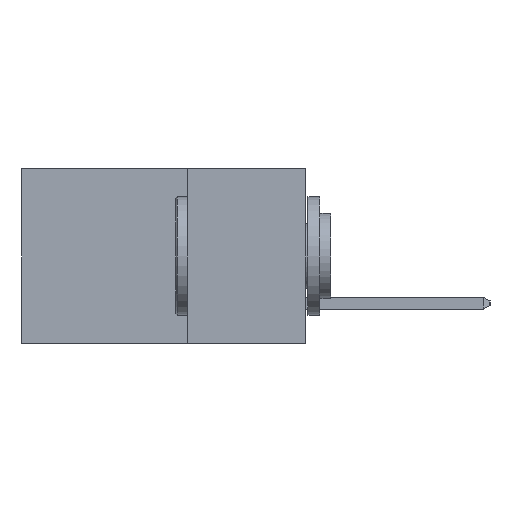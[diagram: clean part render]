
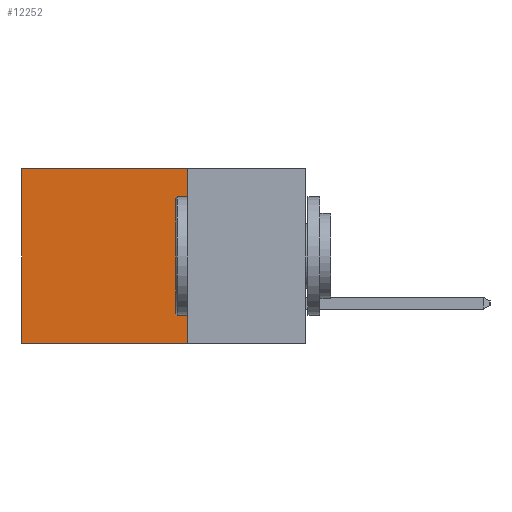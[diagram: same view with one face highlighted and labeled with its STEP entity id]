
A CAD part, left-side view. The second image highlights one B-rep face of the part: STEP entity #12252.
In plain terms, the highlighted planar face has unit normal (-1, 0, 0).
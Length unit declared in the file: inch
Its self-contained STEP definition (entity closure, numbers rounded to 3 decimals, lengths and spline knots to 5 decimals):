
#1746 = VECTOR ( 'NONE', #14443, 39.37008 ) ;
#2975 = VECTOR ( 'NONE', #22714, 39.37008 ) ;
#4077 = EDGE_CURVE ( 'NONE', #5316, #10748, #9700, .T. ) ;
#4194 = VERTEX_POINT ( 'NONE', #17940 ) ;
#4248 = ORIENTED_EDGE ( 'NONE', *, *, #13910, .T. ) ;
#4329 = DIRECTION ( 'NONE',  ( 0., 1., 0. ) ) ;
#4530 = CARTESIAN_POINT ( 'NONE',  ( 0.2615, 0.25, 0. ) ) ;
#4856 = FACE_OUTER_BOUND ( 'NONE', #9946, .T. ) ;
#4945 = VERTEX_POINT ( 'NONE', #9063 ) ;
#5316 = VERTEX_POINT ( 'NONE', #14180 ) ;
#6109 = ORIENTED_EDGE ( 'NONE', *, *, #20372, .F. ) ;
#6473 = LINE ( 'NONE', #19670, #1746 ) ;
#7350 = VECTOR ( 'NONE', #4329, 39.37008 ) ;
#7457 = CARTESIAN_POINT ( 'NONE',  ( 0.2615, 0.6, -0.37 ) ) ;
#9063 = CARTESIAN_POINT ( 'NONE',  ( 0.2615, 0.25, 0. ) ) ;
#9700 = LINE ( 'NONE', #20452, #19223 ) ;
#9946 = EDGE_LOOP ( 'NONE', ( #12433, #6109, #21407, #4248 ) ) ;
#10748 = VERTEX_POINT ( 'NONE', #7457 ) ;
#12191 = LINE ( 'NONE', #4530, #7350 ) ;
#12244 = CARTESIAN_POINT ( 'NONE',  ( 0.2615, 0.25, -0.37 ) ) ;
#12252 = ADVANCED_FACE ( 'NONE', ( #4856 ), #22184, .F. ) ;
#12433 = ORIENTED_EDGE ( 'NONE', *, *, #4077, .T. ) ;
#13910 = EDGE_CURVE ( 'NONE', #4945, #5316, #12191, .T. ) ;
#14180 = CARTESIAN_POINT ( 'NONE',  ( 0.2615, 0.6, 0. ) ) ;
#14443 = DIRECTION ( 'NONE',  ( 0., 0., -1. ) ) ;
#14562 = EDGE_CURVE ( 'NONE', #4945, #4194, #6473, .T. ) ;
#15000 = AXIS2_PLACEMENT_3D ( 'NONE', #22095, #21970, #21949 ) ;
#17940 = CARTESIAN_POINT ( 'NONE',  ( 0.2615, 0.25, -0.37 ) ) ;
#19223 = VECTOR ( 'NONE', #20279, 39.37008 ) ;
#19670 = CARTESIAN_POINT ( 'NONE',  ( 0.2615, 0.25, -0.37 ) ) ;
#20279 = DIRECTION ( 'NONE',  ( 0., 0., -1. ) ) ;
#20372 = EDGE_CURVE ( 'NONE', #4194, #10748, #20843, .T. ) ;
#20452 = CARTESIAN_POINT ( 'NONE',  ( 0.2615, 0.6, -0.37 ) ) ;
#20843 = LINE ( 'NONE', #12244, #2975 ) ;
#21407 = ORIENTED_EDGE ( 'NONE', *, *, #14562, .F. ) ;
#21949 = DIRECTION ( 'NONE',  ( 0., 0., -1. ) ) ;
#21970 = DIRECTION ( 'NONE',  ( 1., 0., 0. ) ) ;
#22095 = CARTESIAN_POINT ( 'NONE',  ( 0.2615, 0.25, -0.37 ) ) ;
#22184 = PLANE ( 'NONE',  #15000 ) ;
#22714 = DIRECTION ( 'NONE',  ( 0., 1., 0. ) ) ;
